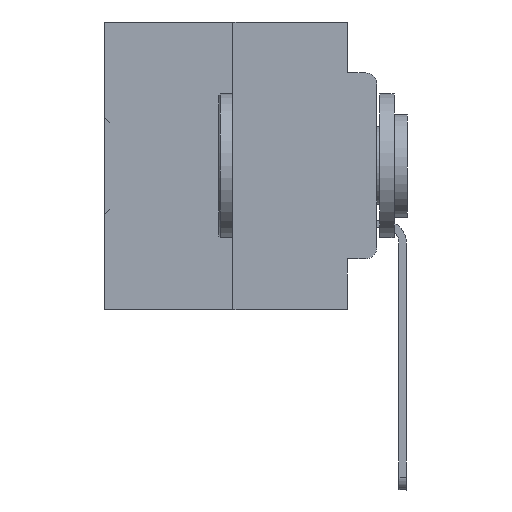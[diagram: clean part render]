
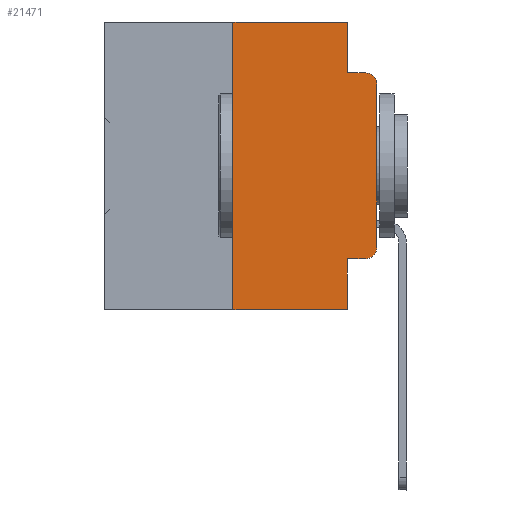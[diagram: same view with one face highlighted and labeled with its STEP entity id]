
A CAD part, left-side view. The second image highlights one B-rep face of the part: STEP entity #21471.
In plain terms, the highlighted planar face has unit normal (-1, 0, 0).
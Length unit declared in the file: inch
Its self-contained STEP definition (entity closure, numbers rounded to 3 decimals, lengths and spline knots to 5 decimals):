
#68 = VECTOR ( 'NONE', #21849, 39.37008 ) ;
#1794 = ORIENTED_EDGE ( 'NONE', *, *, #18392, .F. ) ;
#1966 = DIRECTION ( 'NONE',  ( 0., -1., 0. ) ) ;
#2170 = VECTOR ( 'NONE', #1966, 39.37008 ) ;
#3336 = ORIENTED_EDGE ( 'NONE', *, *, #36541, .T. ) ;
#4374 = FACE_OUTER_BOUND ( 'NONE', #28452, .T. ) ;
#4877 = VERTEX_POINT ( 'NONE', #28855 ) ;
#5048 = LINE ( 'NONE', #23413, #35522 ) ;
#5058 = CARTESIAN_POINT ( 'NONE',  ( 0., 0.051, -0.4115 ) ) ;
#5696 = ORIENTED_EDGE ( 'NONE', *, *, #18070, .F. ) ;
#5974 = ORIENTED_EDGE ( 'NONE', *, *, #8516, .F. ) ;
#6124 = CARTESIAN_POINT ( 'NONE',  ( 0., 0.02, -0.4115 ) ) ;
#6764 = CARTESIAN_POINT ( 'NONE',  ( 0., 0., -0.3915 ) ) ;
#7015 = PLANE ( 'NONE',  #23083 ) ;
#7018 = ORIENTED_EDGE ( 'NONE', *, *, #15587, .F. ) ;
#7250 = CARTESIAN_POINT ( 'NONE',  ( 0., 0.051, 0. ) ) ;
#7661 = LINE ( 'NONE', #30611, #34586 ) ;
#7883 = LINE ( 'NONE', #5058, #29929 ) ;
#8046 = CIRCLE ( 'NONE', #35085, 0.02 ) ;
#8516 = EDGE_CURVE ( 'NONE', #26361, #34695, #7661, .T. ) ;
#8936 = EDGE_CURVE ( 'NONE', #33594, #14850, #36204, .T. ) ;
#9093 = ORIENTED_EDGE ( 'NONE', *, *, #27222, .T. ) ;
#10389 = LINE ( 'NONE', #30322, #68 ) ;
#11325 = CARTESIAN_POINT ( 'NONE',  ( 0., 0.473, -0.5 ) ) ;
#11520 = CARTESIAN_POINT ( 'NONE',  ( 0., 0.02, -0.1085 ) ) ;
#12917 = CARTESIAN_POINT ( 'NONE',  ( 0., 0.02, -0.3915 ) ) ;
#14508 = ORIENTED_EDGE ( 'NONE', *, *, #8936, .T. ) ;
#14850 = VERTEX_POINT ( 'NONE', #28028 ) ;
#15587 = EDGE_CURVE ( 'NONE', #25046, #14850, #33036, .T. ) ;
#16967 = DIRECTION ( 'NONE',  ( -1., 0., 0. ) ) ;
#18030 = CARTESIAN_POINT ( 'NONE',  ( 0., 0.051, 0. ) ) ;
#18070 = EDGE_CURVE ( 'NONE', #34695, #30026, #26148, .T. ) ;
#18392 = EDGE_CURVE ( 'NONE', #33594, #26361, #5048, .T. ) ;
#18640 = VECTOR ( 'NONE', #26333, 39.37008 ) ;
#18667 = CARTESIAN_POINT ( 'NONE',  ( 0., 0.473, 0. ) ) ;
#19374 = DIRECTION ( 'NONE',  ( 0., 0., -1. ) ) ;
#19777 = DIRECTION ( 'NONE',  ( 0., 0., 1. ) ) ;
#19949 = VECTOR ( 'NONE', #19777, 39.37008 ) ;
#20888 = AXIS2_PLACEMENT_3D ( 'NONE', #12917, #24402, #35886 ) ;
#21471 = ADVANCED_FACE ( 'NONE', ( #4374 ), #7015, .F. ) ;
#21849 = DIRECTION ( 'NONE',  ( 0., -1., 0. ) ) ;
#22142 = DIRECTION ( 'NONE',  ( 0., -1., 0. ) ) ;
#22179 = CIRCLE ( 'NONE', #20888, 0.02 ) ;
#22603 = LINE ( 'NONE', #24866, #19949 ) ;
#23083 = AXIS2_PLACEMENT_3D ( 'NONE', #18667, #35612, #19374 ) ;
#23234 = ORIENTED_EDGE ( 'NONE', *, *, #30789, .F. ) ;
#23413 = CARTESIAN_POINT ( 'NONE',  ( 0., 0.25, 0. ) ) ;
#23770 = CARTESIAN_POINT ( 'NONE',  ( 0., 0.051, -0.4115 ) ) ;
#24197 = CARTESIAN_POINT ( 'NONE',  ( 0., 0.25, 0. ) ) ;
#24316 = CARTESIAN_POINT ( 'NONE',  ( 0., 0.051, 0. ) ) ;
#24402 = DIRECTION ( 'NONE',  ( -1., 0., 0. ) ) ;
#24866 = CARTESIAN_POINT ( 'NONE',  ( 0., 0., 0. ) ) ;
#25046 = VERTEX_POINT ( 'NONE', #23770 ) ;
#25199 = DIRECTION ( 'NONE',  ( 0., -1., 0. ) ) ;
#25747 = ORIENTED_EDGE ( 'NONE', *, *, #28197, .T. ) ;
#26148 = LINE ( 'NONE', #18030, #18640 ) ;
#26333 = DIRECTION ( 'NONE',  ( 0., 0., -1. ) ) ;
#26361 = VERTEX_POINT ( 'NONE', #24197 ) ;
#26420 = VERTEX_POINT ( 'NONE', #36055 ) ;
#27222 = EDGE_CURVE ( 'NONE', #31370, #29666, #22179, .T. ) ;
#27613 = ORIENTED_EDGE ( 'NONE', *, *, #31979, .T. ) ;
#28028 = CARTESIAN_POINT ( 'NONE',  ( 0., 0.051, -0.5 ) ) ;
#28197 = EDGE_CURVE ( 'NONE', #25046, #31370, #7883, .T. ) ;
#28452 = EDGE_LOOP ( 'NONE', ( #27613, #3336, #23234, #5696, #5974, #1794, #14508, #7018, #25747, #9093 ) ) ;
#28855 = CARTESIAN_POINT ( 'NONE',  ( 0., 0., -0.1085 ) ) ;
#29666 = VERTEX_POINT ( 'NONE', #6764 ) ;
#29929 = VECTOR ( 'NONE', #25199, 39.37008 ) ;
#30026 = VERTEX_POINT ( 'NONE', #32275 ) ;
#30322 = CARTESIAN_POINT ( 'NONE',  ( 0., 0.051, -0.0885 ) ) ;
#30611 = CARTESIAN_POINT ( 'NONE',  ( 0., 0.473, 0. ) ) ;
#30789 = EDGE_CURVE ( 'NONE', #30026, #26420, #10389, .T. ) ;
#31232 = VECTOR ( 'NONE', #32473, 39.37008 ) ;
#31370 = VERTEX_POINT ( 'NONE', #6124 ) ;
#31602 = CARTESIAN_POINT ( 'NONE',  ( 0., 0.25, -0.5 ) ) ;
#31979 = EDGE_CURVE ( 'NONE', #29666, #4877, #22603, .T. ) ;
#32275 = CARTESIAN_POINT ( 'NONE',  ( 0., 0.051, -0.0885 ) ) ;
#32473 = DIRECTION ( 'NONE',  ( 0., 0., -1. ) ) ;
#33036 = LINE ( 'NONE', #7250, #31232 ) ;
#33594 = VERTEX_POINT ( 'NONE', #31602 ) ;
#33836 = DIRECTION ( 'NONE',  ( 0., 0., 1. ) ) ;
#34586 = VECTOR ( 'NONE', #22142, 39.37008 ) ;
#34650 = DIRECTION ( 'NONE',  ( 0., 0., -1. ) ) ;
#34695 = VERTEX_POINT ( 'NONE', #24316 ) ;
#35085 = AXIS2_PLACEMENT_3D ( 'NONE', #11520, #16967, #34650 ) ;
#35522 = VECTOR ( 'NONE', #33836, 39.37008 ) ;
#35612 = DIRECTION ( 'NONE',  ( 1., 0., 0. ) ) ;
#35886 = DIRECTION ( 'NONE',  ( 0., 0., -1. ) ) ;
#36055 = CARTESIAN_POINT ( 'NONE',  ( 0., 0.02, -0.0885 ) ) ;
#36204 = LINE ( 'NONE', #11325, #2170 ) ;
#36541 = EDGE_CURVE ( 'NONE', #4877, #26420, #8046, .T. ) ;
